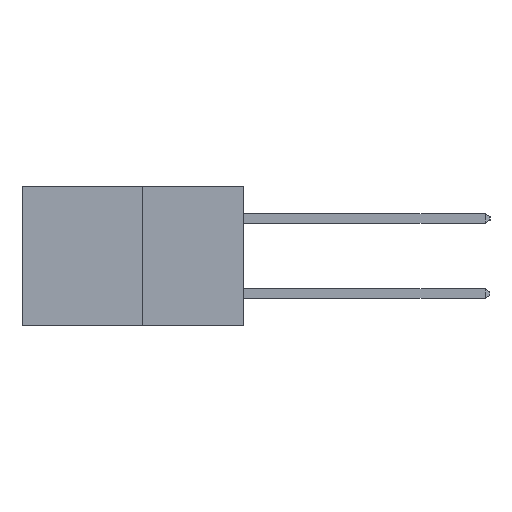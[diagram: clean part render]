
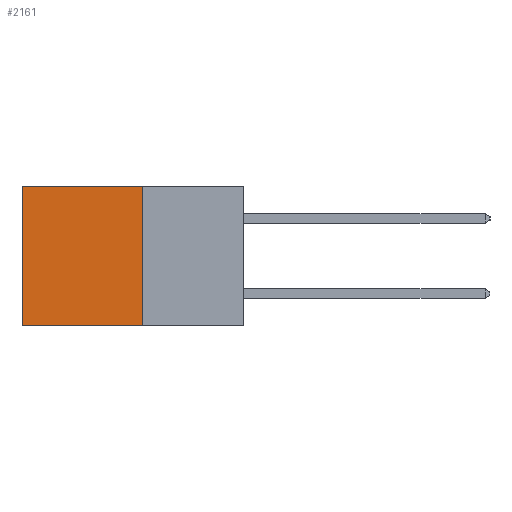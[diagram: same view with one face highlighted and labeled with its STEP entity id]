
A CAD part, left-side view. The second image highlights one B-rep face of the part: STEP entity #2161.
In plain terms, the highlighted planar face has unit normal (-1, 0, 0).
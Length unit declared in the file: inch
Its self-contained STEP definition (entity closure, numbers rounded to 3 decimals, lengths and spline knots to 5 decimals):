
#235 = DIRECTION ( 'NONE',  ( 0., 0., -1. ) ) ;
#272 = DIRECTION ( 'NONE',  ( 1., 0., 0. ) ) ;
#293 = PLANE ( 'NONE',  #3058 ) ;
#843 = CARTESIAN_POINT ( 'NONE',  ( 0.277, 0.27, 0. ) ) ;
#1319 = VECTOR ( 'NONE', #2966, 39.37008 ) ;
#1704 = EDGE_CURVE ( 'NONE', #10271, #5431, #8561, .T. ) ;
#1859 = DIRECTION ( 'NONE',  ( 0., 1., 0. ) ) ;
#1915 = CARTESIAN_POINT ( 'NONE',  ( 0.277, 0.27, 0. ) ) ;
#2161 = ADVANCED_FACE ( 'NONE', ( #7976 ), #293, .F. ) ;
#2365 = VECTOR ( 'NONE', #1859, 39.37008 ) ;
#2417 = ORIENTED_EDGE ( 'NONE', *, *, #1704, .T. ) ;
#2474 = CARTESIAN_POINT ( 'NONE',  ( 0.277, 0.27, -0.37 ) ) ;
#2830 = VERTEX_POINT ( 'NONE', #4657 ) ;
#2926 = CARTESIAN_POINT ( 'NONE',  ( 0.277, 0.27, -0.37 ) ) ;
#2966 = DIRECTION ( 'NONE',  ( 0., 0., -1. ) ) ;
#3058 = AXIS2_PLACEMENT_3D ( 'NONE', #2474, #272, #235 ) ;
#3661 = VECTOR ( 'NONE', #4619, 39.37008 ) ;
#3978 = VERTEX_POINT ( 'NONE', #843 ) ;
#4297 = EDGE_LOOP ( 'NONE', ( #2417, #4961, #7421, #12087 ) ) ;
#4587 = CARTESIAN_POINT ( 'NONE',  ( 0.277, 0.59, -0.37 ) ) ;
#4619 = DIRECTION ( 'NONE',  ( 0., 0., -1. ) ) ;
#4657 = CARTESIAN_POINT ( 'NONE',  ( 0.277, 0.27, -0.37 ) ) ;
#4961 = ORIENTED_EDGE ( 'NONE', *, *, #10111, .F. ) ;
#5431 = VERTEX_POINT ( 'NONE', #6216 ) ;
#6216 = CARTESIAN_POINT ( 'NONE',  ( 0.277, 0.59, -0.37 ) ) ;
#6375 = EDGE_CURVE ( 'NONE', #3978, #10271, #9412, .T. ) ;
#6483 = LINE ( 'NONE', #2926, #1319 ) ;
#7300 = EDGE_CURVE ( 'NONE', #3978, #2830, #6483, .T. ) ;
#7421 = ORIENTED_EDGE ( 'NONE', *, *, #7300, .F. ) ;
#7976 = FACE_OUTER_BOUND ( 'NONE', #4297, .T. ) ;
#8436 = CARTESIAN_POINT ( 'NONE',  ( 0.277, 0.59, 0. ) ) ;
#8561 = LINE ( 'NONE', #4587, #3661 ) ;
#8892 = VECTOR ( 'NONE', #8948, 39.37008 ) ;
#8948 = DIRECTION ( 'NONE',  ( 0., 1., 0. ) ) ;
#9034 = CARTESIAN_POINT ( 'NONE',  ( 0.277, 0.27, -0.37 ) ) ;
#9412 = LINE ( 'NONE', #1915, #2365 ) ;
#10111 = EDGE_CURVE ( 'NONE', #2830, #5431, #11507, .T. ) ;
#10271 = VERTEX_POINT ( 'NONE', #8436 ) ;
#11507 = LINE ( 'NONE', #9034, #8892 ) ;
#12087 = ORIENTED_EDGE ( 'NONE', *, *, #6375, .T. ) ;
